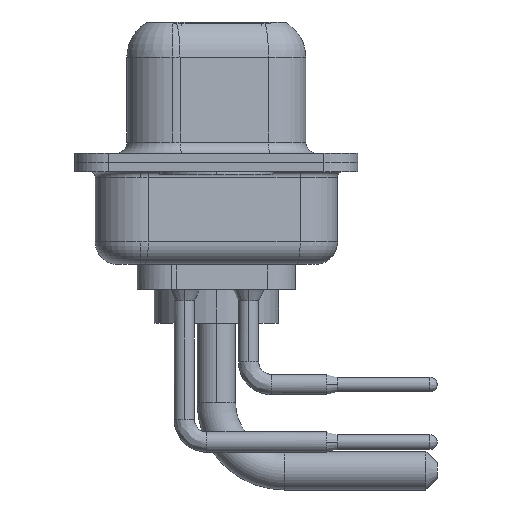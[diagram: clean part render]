
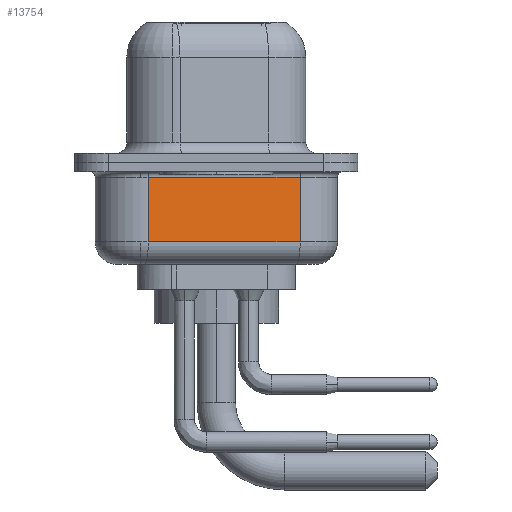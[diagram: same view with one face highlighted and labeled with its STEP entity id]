
A CAD part, left-side view. The second image highlights one B-rep face of the part: STEP entity #13754.
In plain terms, the highlighted planar face has unit normal (-0.985, -0.174, 0).
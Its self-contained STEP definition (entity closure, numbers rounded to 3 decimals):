
#44 = VERTEX_POINT ( 'NONE', #11649 ) ;
#419 = VERTEX_POINT ( 'NONE', #7525 ) ;
#926 = EDGE_LOOP ( 'NONE', ( #5932, #1963, #14302, #7308 ) ) ;
#1512 = VERTEX_POINT ( 'NONE', #13632 ) ;
#1963 = ORIENTED_EDGE ( 'NONE', *, *, #3802, .T. ) ;
#2270 = LINE ( 'NONE', #3386, #10309 ) ;
#2451 = VERTEX_POINT ( 'NONE', #5738 ) ;
#2806 = VECTOR ( 'NONE', #4063, 1000. ) ;
#2975 = CARTESIAN_POINT ( 'NONE',  ( 2.88, 3.003, -4.5 ) ) ;
#3386 = CARTESIAN_POINT ( 'NONE',  ( 2.88, 3.003, -3.5 ) ) ;
#3508 = PLANE ( 'NONE',  #11938 ) ;
#3802 = EDGE_CURVE ( 'NONE', #1512, #2451, #2270, .T. ) ;
#4063 = DIRECTION ( 'NONE',  ( 0., 0., 1. ) ) ;
#4815 = EDGE_CURVE ( 'NONE', #2451, #419, #14022, .T. ) ;
#5738 = CARTESIAN_POINT ( 'NONE',  ( 4.062, -3.697, -3.5 ) ) ;
#5932 = ORIENTED_EDGE ( 'NONE', *, *, #13981, .F. ) ;
#6399 = CARTESIAN_POINT ( 'NONE',  ( 2.88, 3.003, -0.65 ) ) ;
#6507 = DIRECTION ( 'NONE',  ( 0.985, 0.174, 0. ) ) ;
#6650 = FACE_OUTER_BOUND ( 'NONE', #926, .T. ) ;
#7304 = DIRECTION ( 'NONE',  ( -0.174, 0.985, 0. ) ) ;
#7308 = ORIENTED_EDGE ( 'NONE', *, *, #11576, .T. ) ;
#7525 = CARTESIAN_POINT ( 'NONE',  ( 4.062, -3.697, -0.65 ) ) ;
#7992 = CARTESIAN_POINT ( 'NONE',  ( 2.88, 3.003, -4.5 ) ) ;
#8745 = DIRECTION ( 'NONE',  ( 0.174, -0.985, 0. ) ) ;
#10309 = VECTOR ( 'NONE', #8745, 1000. ) ;
#10600 = LINE ( 'NONE', #2975, #12185 ) ;
#10864 = CARTESIAN_POINT ( 'NONE',  ( 4.062, -3.697, -4.5 ) ) ;
#10975 = DIRECTION ( 'NONE',  ( -0.174, 0.985, 0. ) ) ;
#11576 = EDGE_CURVE ( 'NONE', #419, #44, #14179, .T. ) ;
#11649 = CARTESIAN_POINT ( 'NONE',  ( 2.88, 3.003, -0.65 ) ) ;
#11904 = DIRECTION ( 'NONE',  ( 0., 0., 1. ) ) ;
#11938 = AXIS2_PLACEMENT_3D ( 'NONE', #7992, #6507, #10975 ) ;
#12185 = VECTOR ( 'NONE', #11904, 1000. ) ;
#13632 = CARTESIAN_POINT ( 'NONE',  ( 2.88, 3.003, -3.5 ) ) ;
#13754 = ADVANCED_FACE ( 'NONE', ( #6650 ), #3508, .F. ) ;
#13831 = VECTOR ( 'NONE', #7304, 1000. ) ;
#13981 = EDGE_CURVE ( 'NONE', #1512, #44, #10600, .T. ) ;
#14022 = LINE ( 'NONE', #10864, #2806 ) ;
#14179 = LINE ( 'NONE', #6399, #13831 ) ;
#14302 = ORIENTED_EDGE ( 'NONE', *, *, #4815, .T. ) ;
